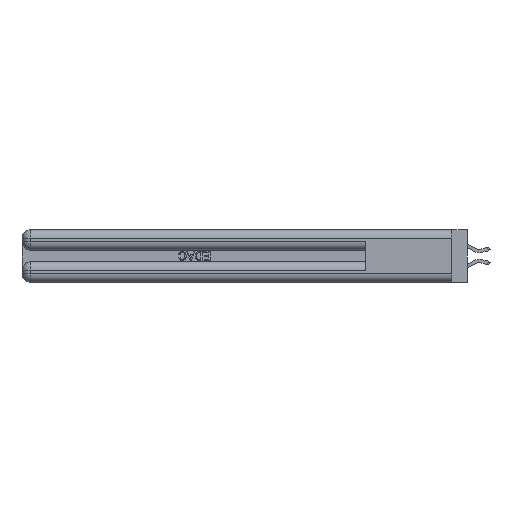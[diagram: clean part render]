
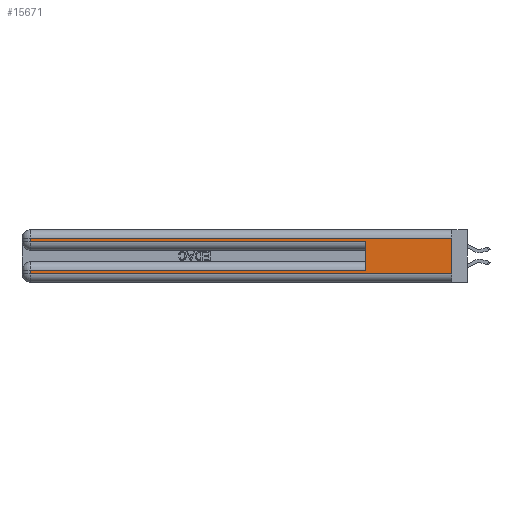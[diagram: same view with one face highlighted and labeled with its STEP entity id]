
A CAD part, left-side view. The second image highlights one B-rep face of the part: STEP entity #15671.
In plain terms, the highlighted planar face has unit normal (-1, 0, 0).
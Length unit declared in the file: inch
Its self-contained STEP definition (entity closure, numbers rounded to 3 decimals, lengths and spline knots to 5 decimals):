
#198 = EDGE_LOOP ( 'NONE', ( #3763, #31244, #33986, #6065, #41144, #5923, #33479, #22141 ) ) ;
#254 = DIRECTION ( 'NONE',  ( 0., -1., 0. ) ) ;
#347 = LINE ( 'NONE', #27754, #26593 ) ;
#1658 = CARTESIAN_POINT ( 'NONE',  ( 0., 2.94, 0.085 ) ) ;
#2275 = CARTESIAN_POINT ( 'NONE',  ( 0., 0.6, 0.285 ) ) ;
#2543 = CARTESIAN_POINT ( 'NONE',  ( 0., 2.94, 0.31 ) ) ;
#2835 = LINE ( 'NONE', #32200, #20307 ) ;
#3096 = DIRECTION ( 'NONE',  ( 0., 0., -1. ) ) ;
#3395 = LINE ( 'NONE', #9260, #19833 ) ;
#3473 = LINE ( 'NONE', #17961, #37259 ) ;
#3763 = ORIENTED_EDGE ( 'NONE', *, *, #36889, .F. ) ;
#5923 = ORIENTED_EDGE ( 'NONE', *, *, #32580, .T. ) ;
#6065 = ORIENTED_EDGE ( 'NONE', *, *, #23725, .T. ) ;
#6979 = CARTESIAN_POINT ( 'NONE',  ( 0., 0., 0.285 ) ) ;
#7171 = EDGE_CURVE ( 'NONE', #21958, #34556, #10637, .T. ) ;
#8337 = EDGE_CURVE ( 'NONE', #18981, #21958, #2835, .T. ) ;
#9260 = CARTESIAN_POINT ( 'NONE',  ( 0., 0., 0.31 ) ) ;
#9586 = DIRECTION ( 'NONE',  ( 0., 0., -1. ) ) ;
#10526 = VECTOR ( 'NONE', #38766, 39.37008 ) ;
#10637 = LINE ( 'NONE', #16758, #25928 ) ;
#11559 = LINE ( 'NONE', #12709, #10526 ) ;
#12042 = EDGE_CURVE ( 'NONE', #22424, #22301, #347, .T. ) ;
#12676 = DIRECTION ( 'NONE',  ( 0., 0., -1. ) ) ;
#12709 = CARTESIAN_POINT ( 'NONE',  ( 0., 0., 0.085 ) ) ;
#13406 = CARTESIAN_POINT ( 'NONE',  ( 0., 0.6, 0.085 ) ) ;
#14315 = EDGE_CURVE ( 'NONE', #29025, #31281, #3395, .T. ) ;
#14668 = DIRECTION ( 'NONE',  ( 0., 0., 1. ) ) ;
#15531 = VECTOR ( 'NONE', #9586, 39.37008 ) ;
#15671 = ADVANCED_FACE ( 'NONE', ( #19715 ), #35715, .F. ) ;
#15838 = DIRECTION ( 'NONE',  ( 0., 1., 0. ) ) ;
#16333 = VERTEX_POINT ( 'NONE', #16987 ) ;
#16384 = CARTESIAN_POINT ( 'NONE',  ( 0., 0., 0.31 ) ) ;
#16758 = CARTESIAN_POINT ( 'NONE',  ( 0., 0., 0.06 ) ) ;
#16987 = CARTESIAN_POINT ( 'NONE',  ( 0., 2.94, 0.285 ) ) ;
#17914 = EDGE_CURVE ( 'NONE', #31281, #16333, #23184, .T. ) ;
#17961 = CARTESIAN_POINT ( 'NONE',  ( 0., 0., 0.37 ) ) ;
#18981 = VERTEX_POINT ( 'NONE', #1658 ) ;
#19715 = FACE_OUTER_BOUND ( 'NONE', #198, .T. ) ;
#19833 = VECTOR ( 'NONE', #15838, 39.37008 ) ;
#20307 = VECTOR ( 'NONE', #12676, 39.37008 ) ;
#21233 = DIRECTION ( 'NONE',  ( 0., 0., -1. ) ) ;
#21958 = VERTEX_POINT ( 'NONE', #33364 ) ;
#22141 = ORIENTED_EDGE ( 'NONE', *, *, #7171, .T. ) ;
#22301 = VERTEX_POINT ( 'NONE', #2275 ) ;
#22424 = VERTEX_POINT ( 'NONE', #13406 ) ;
#22766 = DIRECTION ( 'NONE',  ( 1., 0., 0. ) ) ;
#23184 = LINE ( 'NONE', #25842, #15531 ) ;
#23725 = EDGE_CURVE ( 'NONE', #16333, #22301, #41943, .T. ) ;
#25842 = CARTESIAN_POINT ( 'NONE',  ( 0., 2.94, 0.37 ) ) ;
#25928 = VECTOR ( 'NONE', #254, 39.37008 ) ;
#26593 = VECTOR ( 'NONE', #14668, 39.37008 ) ;
#27754 = CARTESIAN_POINT ( 'NONE',  ( 0., 0.6, 0.145 ) ) ;
#29025 = VERTEX_POINT ( 'NONE', #16384 ) ;
#29991 = DIRECTION ( 'NONE',  ( 0., -1., 0. ) ) ;
#31058 = AXIS2_PLACEMENT_3D ( 'NONE', #42195, #22766, #3096 ) ;
#31244 = ORIENTED_EDGE ( 'NONE', *, *, #14315, .T. ) ;
#31281 = VERTEX_POINT ( 'NONE', #2543 ) ;
#32200 = CARTESIAN_POINT ( 'NONE',  ( 0., 2.94, 0.37 ) ) ;
#32580 = EDGE_CURVE ( 'NONE', #22424, #18981, #11559, .T. ) ;
#33338 = VECTOR ( 'NONE', #29991, 39.37008 ) ;
#33364 = CARTESIAN_POINT ( 'NONE',  ( 0., 2.94, 0.06 ) ) ;
#33479 = ORIENTED_EDGE ( 'NONE', *, *, #8337, .T. ) ;
#33986 = ORIENTED_EDGE ( 'NONE', *, *, #17914, .T. ) ;
#34556 = VERTEX_POINT ( 'NONE', #36034 ) ;
#35715 = PLANE ( 'NONE',  #31058 ) ;
#36034 = CARTESIAN_POINT ( 'NONE',  ( 0., 0., 0.06 ) ) ;
#36889 = EDGE_CURVE ( 'NONE', #29025, #34556, #3473, .T. ) ;
#37259 = VECTOR ( 'NONE', #21233, 39.37008 ) ;
#38766 = DIRECTION ( 'NONE',  ( 0., 1., 0. ) ) ;
#41144 = ORIENTED_EDGE ( 'NONE', *, *, #12042, .F. ) ;
#41943 = LINE ( 'NONE', #6979, #33338 ) ;
#42195 = CARTESIAN_POINT ( 'NONE',  ( 0., 0., 0.37 ) ) ;
